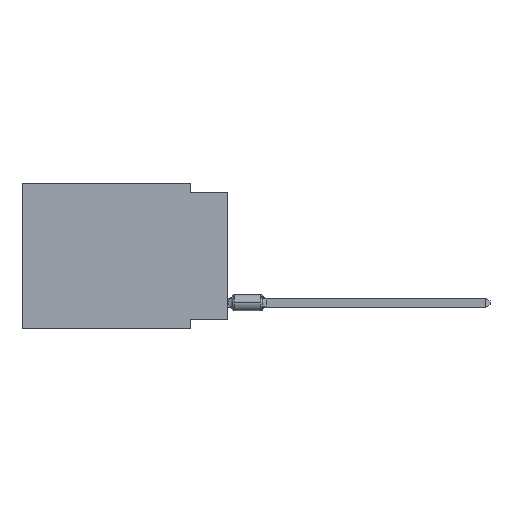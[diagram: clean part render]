
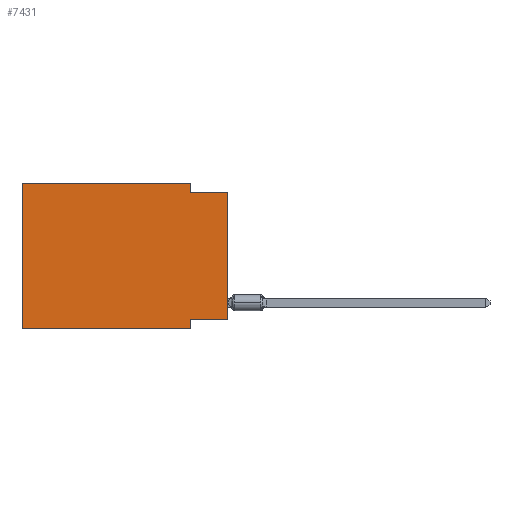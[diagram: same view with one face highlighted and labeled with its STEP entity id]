
A CAD part, left-side view. The second image highlights one B-rep face of the part: STEP entity #7431.
In plain terms, the highlighted planar face has unit normal (-1, 0, 0).
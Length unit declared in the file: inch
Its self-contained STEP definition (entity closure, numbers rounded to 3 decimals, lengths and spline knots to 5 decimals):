
#59 = DIRECTION ( 'NONE',  ( 0., -1., 0. ) ) ;
#195 = EDGE_CURVE ( 'NONE', #5987, #5550, #5109, .T. ) ;
#456 = VERTEX_POINT ( 'NONE', #12485 ) ;
#627 = CARTESIAN_POINT ( 'NONE',  ( 0., 0.1, -0.39 ) ) ;
#1031 = VECTOR ( 'NONE', #9126, 39.37008 ) ;
#1308 = CARTESIAN_POINT ( 'NONE',  ( 0., 0.1, 0. ) ) ;
#1345 = EDGE_LOOP ( 'NONE', ( #6146, #13141, #8562, #7941, #7036, #8507, #2701, #1703 ) ) ;
#1592 = FACE_OUTER_BOUND ( 'NONE', #1345, .T. ) ;
#1703 = ORIENTED_EDGE ( 'NONE', *, *, #11440, .F. ) ;
#1845 = CARTESIAN_POINT ( 'NONE',  ( 0., 0.1, -0.025 ) ) ;
#1867 = EDGE_CURVE ( 'NONE', #9638, #5550, #2227, .T. ) ;
#1985 = AXIS2_PLACEMENT_3D ( 'NONE', #13561, #3729, #8111 ) ;
#2115 = DIRECTION ( 'NONE',  ( 0., 0., -1. ) ) ;
#2158 = VERTEX_POINT ( 'NONE', #4073 ) ;
#2227 = LINE ( 'NONE', #9892, #5668 ) ;
#2331 = CARTESIAN_POINT ( 'NONE',  ( 0., 0., -0.365 ) ) ;
#2701 = ORIENTED_EDGE ( 'NONE', *, *, #4740, .F. ) ;
#2862 = EDGE_CURVE ( 'NONE', #456, #2158, #7828, .T. ) ;
#3107 = DIRECTION ( 'NONE',  ( 0., 1., 0. ) ) ;
#3299 = DIRECTION ( 'NONE',  ( 0., -1., 0. ) ) ;
#3691 = VERTEX_POINT ( 'NONE', #13293 ) ;
#3729 = DIRECTION ( 'NONE',  ( 1., 0., 0. ) ) ;
#4073 = CARTESIAN_POINT ( 'NONE',  ( 0., 0.1, 0. ) ) ;
#4630 = VERTEX_POINT ( 'NONE', #12456 ) ;
#4740 = EDGE_CURVE ( 'NONE', #4630, #3691, #13810, .T. ) ;
#5109 = LINE ( 'NONE', #12872, #7209 ) ;
#5269 = CARTESIAN_POINT ( 'NONE',  ( 0., 0., -0.365 ) ) ;
#5550 = VERTEX_POINT ( 'NONE', #9532 ) ;
#5668 = VECTOR ( 'NONE', #7820, 39.37008 ) ;
#5879 = VECTOR ( 'NONE', #2115, 39.37008 ) ;
#5889 = PLANE ( 'NONE',  #1985 ) ;
#5987 = VERTEX_POINT ( 'NONE', #1845 ) ;
#6146 = ORIENTED_EDGE ( 'NONE', *, *, #1867, .T. ) ;
#6366 = DIRECTION ( 'NONE',  ( 0., 0., -1. ) ) ;
#6370 = VECTOR ( 'NONE', #3107, 39.37008 ) ;
#6434 = EDGE_CURVE ( 'NONE', #7500, #456, #8426, .T. ) ;
#6475 = DIRECTION ( 'NONE',  ( 0., -1., 0. ) ) ;
#6604 = CARTESIAN_POINT ( 'NONE',  ( 0., 0.55, 0. ) ) ;
#6657 = LINE ( 'NONE', #11168, #8215 ) ;
#7036 = ORIENTED_EDGE ( 'NONE', *, *, #6434, .F. ) ;
#7209 = VECTOR ( 'NONE', #6475, 39.37008 ) ;
#7431 = ADVANCED_FACE ( 'NONE', ( #1592 ), #5889, .F. ) ;
#7500 = VERTEX_POINT ( 'NONE', #8393 ) ;
#7570 = LINE ( 'NONE', #5269, #6370 ) ;
#7820 = DIRECTION ( 'NONE',  ( 0., 0., 1. ) ) ;
#7828 = LINE ( 'NONE', #6604, #8209 ) ;
#7941 = ORIENTED_EDGE ( 'NONE', *, *, #2862, .F. ) ;
#8111 = DIRECTION ( 'NONE',  ( 0., 0., -1. ) ) ;
#8209 = VECTOR ( 'NONE', #3299, 39.37008 ) ;
#8215 = VECTOR ( 'NONE', #59, 39.37008 ) ;
#8393 = CARTESIAN_POINT ( 'NONE',  ( 0., 0.55, -0.39 ) ) ;
#8426 = LINE ( 'NONE', #12425, #1031 ) ;
#8507 = ORIENTED_EDGE ( 'NONE', *, *, #12459, .T. ) ;
#8562 = ORIENTED_EDGE ( 'NONE', *, *, #10038, .F. ) ;
#9126 = DIRECTION ( 'NONE',  ( 0., 0., 1. ) ) ;
#9532 = CARTESIAN_POINT ( 'NONE',  ( 0., 0., -0.025 ) ) ;
#9638 = VERTEX_POINT ( 'NONE', #2331 ) ;
#9892 = CARTESIAN_POINT ( 'NONE',  ( 0., 0., 0. ) ) ;
#10038 = EDGE_CURVE ( 'NONE', #2158, #5987, #11998, .T. ) ;
#11168 = CARTESIAN_POINT ( 'NONE',  ( 0., 0.55, -0.39 ) ) ;
#11440 = EDGE_CURVE ( 'NONE', #9638, #4630, #7570, .T. ) ;
#11998 = LINE ( 'NONE', #1308, #5879 ) ;
#12382 = VECTOR ( 'NONE', #6366, 39.37008 ) ;
#12425 = CARTESIAN_POINT ( 'NONE',  ( 0., 0.55, 0. ) ) ;
#12456 = CARTESIAN_POINT ( 'NONE',  ( 0., 0.1, -0.365 ) ) ;
#12459 = EDGE_CURVE ( 'NONE', #7500, #3691, #6657, .T. ) ;
#12485 = CARTESIAN_POINT ( 'NONE',  ( 0., 0.55, 0. ) ) ;
#12872 = CARTESIAN_POINT ( 'NONE',  ( 0., 0., -0.025 ) ) ;
#13141 = ORIENTED_EDGE ( 'NONE', *, *, #195, .F. ) ;
#13293 = CARTESIAN_POINT ( 'NONE',  ( 0., 0.1, -0.39 ) ) ;
#13561 = CARTESIAN_POINT ( 'NONE',  ( 0., 0.55, 0. ) ) ;
#13810 = LINE ( 'NONE', #627, #12382 ) ;
